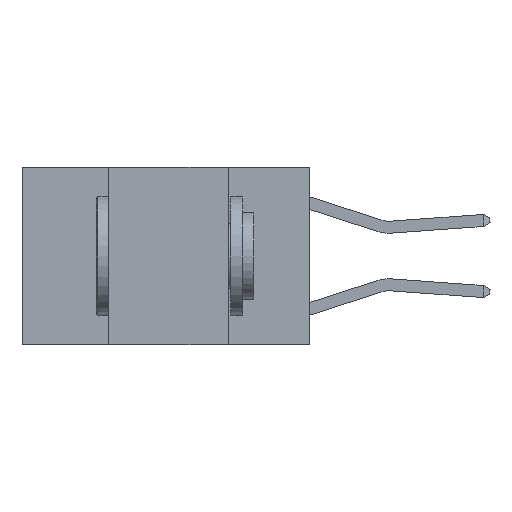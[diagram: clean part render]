
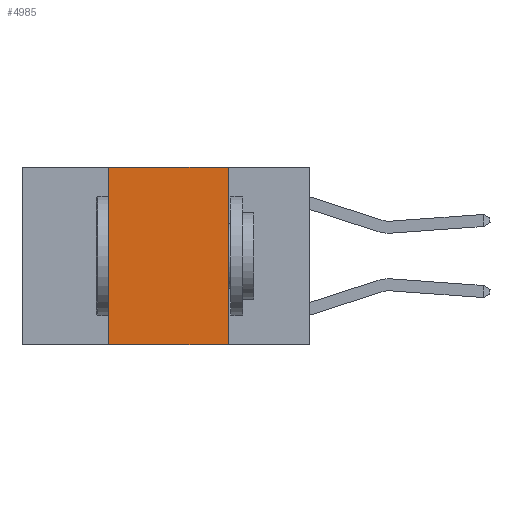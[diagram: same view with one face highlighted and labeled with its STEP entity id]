
A CAD part, left-side view. The second image highlights one B-rep face of the part: STEP entity #4985.
In plain terms, the highlighted planar face has unit normal (-1, 0, 0).
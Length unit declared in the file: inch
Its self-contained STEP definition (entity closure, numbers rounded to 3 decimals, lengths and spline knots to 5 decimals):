
#494 = LINE ( 'NONE', #17182, #14906 ) ;
#556 = CARTESIAN_POINT ( 'NONE',  ( 0., 0.6, 0. ) ) ;
#665 = EDGE_CURVE ( 'NONE', #2997, #7266, #494, .T. ) ;
#1011 = DIRECTION ( 'NONE',  ( 0., -1., 0. ) ) ;
#1548 = VECTOR ( 'NONE', #14994, 39.37008 ) ;
#2997 = VERTEX_POINT ( 'NONE', #23296 ) ;
#3607 = EDGE_LOOP ( 'NONE', ( #12169, #19986, #24430, #4408 ) ) ;
#4408 = ORIENTED_EDGE ( 'NONE', *, *, #20476, .T. ) ;
#4985 = ADVANCED_FACE ( 'NONE', ( #17283 ), #11289, .F. ) ;
#5282 = VERTEX_POINT ( 'NONE', #7384 ) ;
#5332 = AXIS2_PLACEMENT_3D ( 'NONE', #556, #9419, #17156 ) ;
#5612 = CARTESIAN_POINT ( 'NONE',  ( 0., 0.6, -0.37 ) ) ;
#7250 = LINE ( 'NONE', #5612, #1548 ) ;
#7266 = VERTEX_POINT ( 'NONE', #9471 ) ;
#7384 = CARTESIAN_POINT ( 'NONE',  ( 0., 0.17, -0.37 ) ) ;
#7566 = EDGE_CURVE ( 'NONE', #7266, #21480, #22176, .T. ) ;
#7645 = CARTESIAN_POINT ( 'NONE',  ( 0., 0.17, 0. ) ) ;
#8072 = DIRECTION ( 'NONE',  ( 0., 0., 1. ) ) ;
#9362 = EDGE_CURVE ( 'NONE', #21480, #5282, #13808, .T. ) ;
#9419 = DIRECTION ( 'NONE',  ( 1., 0., 0. ) ) ;
#9471 = CARTESIAN_POINT ( 'NONE',  ( 0., 0.42, 0. ) ) ;
#10049 = DIRECTION ( 'NONE',  ( 0., 0., -1. ) ) ;
#11289 = PLANE ( 'NONE',  #5332 ) ;
#12031 = VECTOR ( 'NONE', #10049, 39.37008 ) ;
#12169 = ORIENTED_EDGE ( 'NONE', *, *, #9362, .F. ) ;
#12586 = VECTOR ( 'NONE', #1011, 39.37008 ) ;
#13808 = LINE ( 'NONE', #21412, #12031 ) ;
#14906 = VECTOR ( 'NONE', #8072, 39.37008 ) ;
#14994 = DIRECTION ( 'NONE',  ( 0., -1., 0. ) ) ;
#17156 = DIRECTION ( 'NONE',  ( 0., 0., -1. ) ) ;
#17182 = CARTESIAN_POINT ( 'NONE',  ( 0., 0.42, 0. ) ) ;
#17283 = FACE_OUTER_BOUND ( 'NONE', #3607, .T. ) ;
#19986 = ORIENTED_EDGE ( 'NONE', *, *, #7566, .F. ) ;
#20038 = CARTESIAN_POINT ( 'NONE',  ( 0., 0.6, 0. ) ) ;
#20476 = EDGE_CURVE ( 'NONE', #2997, #5282, #7250, .T. ) ;
#21412 = CARTESIAN_POINT ( 'NONE',  ( 0., 0.17, 0. ) ) ;
#21480 = VERTEX_POINT ( 'NONE', #7645 ) ;
#22176 = LINE ( 'NONE', #20038, #12586 ) ;
#23296 = CARTESIAN_POINT ( 'NONE',  ( 0., 0.42, -0.37 ) ) ;
#24430 = ORIENTED_EDGE ( 'NONE', *, *, #665, .F. ) ;
